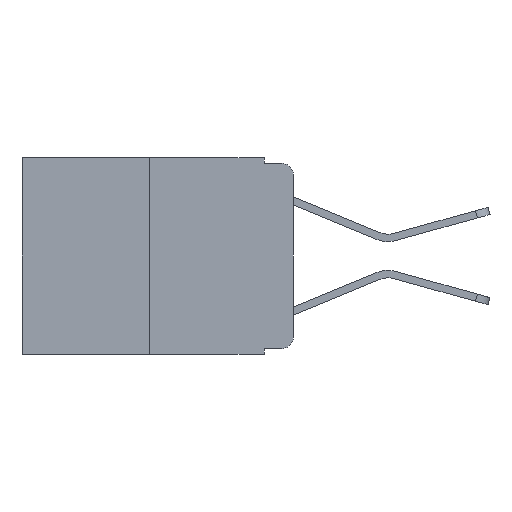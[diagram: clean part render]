
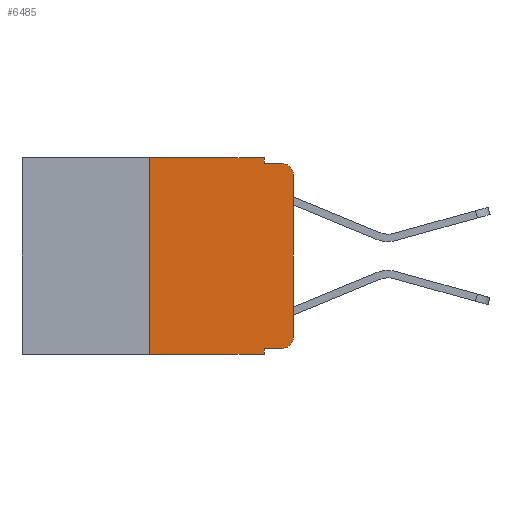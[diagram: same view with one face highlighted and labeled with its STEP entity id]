
A CAD part, left-side view. The second image highlights one B-rep face of the part: STEP entity #6485.
In plain terms, the highlighted planar face has unit normal (-1, 0, 0).
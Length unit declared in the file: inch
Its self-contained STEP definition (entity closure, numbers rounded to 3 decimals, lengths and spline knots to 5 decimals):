
#37 = DIRECTION ( 'NONE',  ( 0., 0., 1. ) ) ;
#139 = EDGE_CURVE ( 'NONE', #3058, #2541, #10469, .T. ) ;
#451 = VERTEX_POINT ( 'NONE', #10428 ) ;
#537 = CARTESIAN_POINT ( 'NONE',  ( 0., 0.051, -0.343 ) ) ;
#645 = LINE ( 'NONE', #6741, #8753 ) ;
#727 = DIRECTION ( 'NONE',  ( 0., -1., 0. ) ) ;
#735 = EDGE_CURVE ( 'NONE', #2541, #7750, #2547, .T. ) ;
#874 = CARTESIAN_POINT ( 'NONE',  ( 0., 0.051, -0.333 ) ) ;
#900 = AXIS2_PLACEMENT_3D ( 'NONE', #5971, #6400, #6328 ) ;
#962 = CARTESIAN_POINT ( 'NONE',  ( 0., 0.25, 0. ) ) ;
#983 = VECTOR ( 'NONE', #727, 39.37008 ) ;
#1037 = CARTESIAN_POINT ( 'NONE',  ( 0., 0.051, 0. ) ) ;
#1567 = EDGE_LOOP ( 'NONE', ( #8648, #7439, #8211, #7811, #9792, #5900, #10535, #3951, #2425, #3299 ) ) ;
#1609 = VERTEX_POINT ( 'NONE', #537 ) ;
#1867 = CARTESIAN_POINT ( 'NONE',  ( 0., 0.473, 0. ) ) ;
#1929 = LINE ( 'NONE', #5202, #3483 ) ;
#2072 = LINE ( 'NONE', #2157, #8587 ) ;
#2157 = CARTESIAN_POINT ( 'NONE',  ( 0., 0.051, -0.01 ) ) ;
#2168 = FACE_OUTER_BOUND ( 'NONE', #1567, .T. ) ;
#2176 = VERTEX_POINT ( 'NONE', #1037 ) ;
#2181 = VERTEX_POINT ( 'NONE', #6809 ) ;
#2425 = ORIENTED_EDGE ( 'NONE', *, *, #5831, .T. ) ;
#2526 = CARTESIAN_POINT ( 'NONE',  ( 0., 0., 0. ) ) ;
#2541 = VERTEX_POINT ( 'NONE', #6343 ) ;
#2547 = CIRCLE ( 'NONE', #900, 0.02 ) ;
#2619 = VECTOR ( 'NONE', #9336, 39.37008 ) ;
#2626 = EDGE_CURVE ( 'NONE', #2181, #7750, #2072, .T. ) ;
#2781 = DIRECTION ( 'NONE',  ( 1., 0., 0. ) ) ;
#3058 = VERTEX_POINT ( 'NONE', #4551 ) ;
#3133 = AXIS2_PLACEMENT_3D ( 'NONE', #1867, #2781, #8436 ) ;
#3299 = ORIENTED_EDGE ( 'NONE', *, *, #6395, .T. ) ;
#3480 = CARTESIAN_POINT ( 'NONE',  ( 0., 0.473, -0.343 ) ) ;
#3483 = VECTOR ( 'NONE', #5227, 39.37008 ) ;
#3686 = DIRECTION ( 'NONE',  ( 0., -1., 0. ) ) ;
#3786 = EDGE_CURVE ( 'NONE', #2176, #2181, #1929, .T. ) ;
#3951 = ORIENTED_EDGE ( 'NONE', *, *, #5320, .F. ) ;
#4062 = VECTOR ( 'NONE', #3686, 39.37008 ) ;
#4301 = EDGE_CURVE ( 'NONE', #5996, #5857, #9067, .T. ) ;
#4325 = VECTOR ( 'NONE', #7234, 39.37008 ) ;
#4349 = DIRECTION ( 'NONE',  ( -1., 0., 0. ) ) ;
#4530 = CARTESIAN_POINT ( 'NONE',  ( 0., 0.051, 0. ) ) ;
#4551 = CARTESIAN_POINT ( 'NONE',  ( 0., 0., -0.313 ) ) ;
#5016 = LINE ( 'NONE', #4530, #2619 ) ;
#5112 = CIRCLE ( 'NONE', #7589, 0.02 ) ;
#5202 = CARTESIAN_POINT ( 'NONE',  ( 0., 0.051, 0. ) ) ;
#5227 = DIRECTION ( 'NONE',  ( 0., 0., -1. ) ) ;
#5257 = LINE ( 'NONE', #3480, #983 ) ;
#5320 = EDGE_CURVE ( 'NONE', #7740, #1609, #5016, .T. ) ;
#5710 = EDGE_CURVE ( 'NONE', #5996, #1609, #5257, .T. ) ;
#5831 = EDGE_CURVE ( 'NONE', #7740, #451, #6867, .T. ) ;
#5857 = VERTEX_POINT ( 'NONE', #962 ) ;
#5900 = ORIENTED_EDGE ( 'NONE', *, *, #4301, .F. ) ;
#5971 = CARTESIAN_POINT ( 'NONE',  ( 0., 0.02, -0.03 ) ) ;
#5996 = VERTEX_POINT ( 'NONE', #10210 ) ;
#6209 = VECTOR ( 'NONE', #37, 39.37008 ) ;
#6328 = DIRECTION ( 'NONE',  ( 0., 0., -1. ) ) ;
#6343 = CARTESIAN_POINT ( 'NONE',  ( 0., 0., -0.03 ) ) ;
#6395 = EDGE_CURVE ( 'NONE', #451, #3058, #5112, .T. ) ;
#6400 = DIRECTION ( 'NONE',  ( -1., 0., 0. ) ) ;
#6485 = ADVANCED_FACE ( 'NONE', ( #2168 ), #6769, .F. ) ;
#6554 = CARTESIAN_POINT ( 'NONE',  ( 0., 0.051, -0.333 ) ) ;
#6741 = CARTESIAN_POINT ( 'NONE',  ( 0., 0.473, 0. ) ) ;
#6769 = PLANE ( 'NONE',  #3133 ) ;
#6809 = CARTESIAN_POINT ( 'NONE',  ( 0., 0.051, -0.01 ) ) ;
#6867 = LINE ( 'NONE', #874, #4062 ) ;
#7234 = DIRECTION ( 'NONE',  ( 0., 0., 1. ) ) ;
#7355 = CARTESIAN_POINT ( 'NONE',  ( 0., 0.02, -0.01 ) ) ;
#7439 = ORIENTED_EDGE ( 'NONE', *, *, #735, .T. ) ;
#7568 = DIRECTION ( 'NONE',  ( 0., -1., 0. ) ) ;
#7589 = AXIS2_PLACEMENT_3D ( 'NONE', #9129, #4349, #9922 ) ;
#7706 = DIRECTION ( 'NONE',  ( 0., -1., 0. ) ) ;
#7740 = VERTEX_POINT ( 'NONE', #6554 ) ;
#7750 = VERTEX_POINT ( 'NONE', #7355 ) ;
#7811 = ORIENTED_EDGE ( 'NONE', *, *, #3786, .F. ) ;
#8211 = ORIENTED_EDGE ( 'NONE', *, *, #2626, .F. ) ;
#8436 = DIRECTION ( 'NONE',  ( 0., 0., -1. ) ) ;
#8587 = VECTOR ( 'NONE', #7706, 39.37008 ) ;
#8648 = ORIENTED_EDGE ( 'NONE', *, *, #139, .T. ) ;
#8753 = VECTOR ( 'NONE', #7568, 39.37008 ) ;
#8858 = CARTESIAN_POINT ( 'NONE',  ( 0., 0.25, 0. ) ) ;
#9067 = LINE ( 'NONE', #8858, #4325 ) ;
#9129 = CARTESIAN_POINT ( 'NONE',  ( 0., 0.02, -0.313 ) ) ;
#9336 = DIRECTION ( 'NONE',  ( 0., 0., -1. ) ) ;
#9792 = ORIENTED_EDGE ( 'NONE', *, *, #10305, .F. ) ;
#9922 = DIRECTION ( 'NONE',  ( 0., 0., -1. ) ) ;
#10210 = CARTESIAN_POINT ( 'NONE',  ( 0., 0.25, -0.343 ) ) ;
#10305 = EDGE_CURVE ( 'NONE', #5857, #2176, #645, .T. ) ;
#10428 = CARTESIAN_POINT ( 'NONE',  ( 0., 0.02, -0.333 ) ) ;
#10469 = LINE ( 'NONE', #2526, #6209 ) ;
#10535 = ORIENTED_EDGE ( 'NONE', *, *, #5710, .T. ) ;
